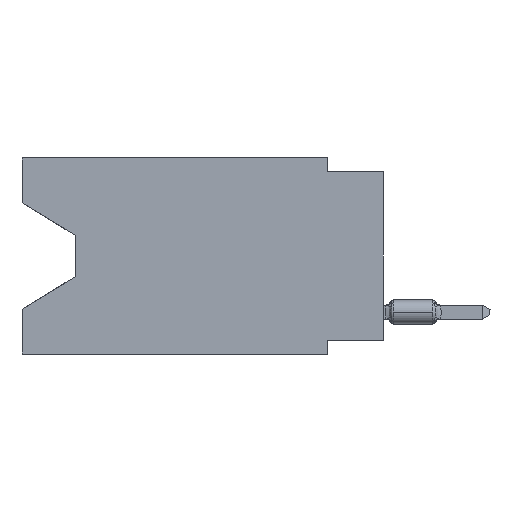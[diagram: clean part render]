
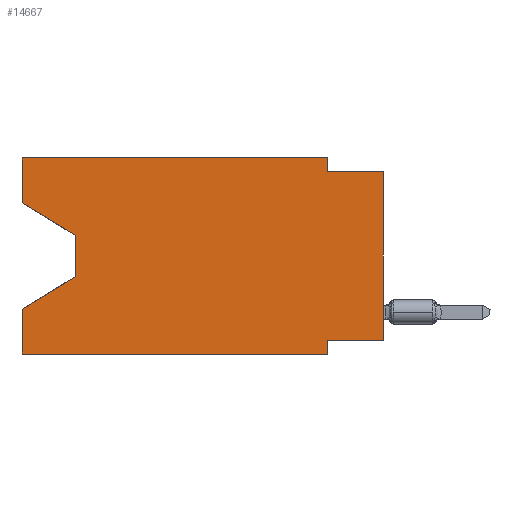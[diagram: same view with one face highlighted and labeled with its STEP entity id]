
A CAD part, left-side view. The second image highlights one B-rep face of the part: STEP entity #14667.
In plain terms, the highlighted planar face has unit normal (-1, 0, 0).
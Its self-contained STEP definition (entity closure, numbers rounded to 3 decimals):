
#1926 = EDGE_CURVE ( 'NONE', #49698, #31826, #39422, .T. ) ;
#3061 = EDGE_CURVE ( 'NONE', #45013, #55166, #20508, .T. ) ;
#3267 = VECTOR ( 'NONE', #7442, 1000. ) ;
#3288 = CARTESIAN_POINT ( 'NONE',  ( 0., 16.383, -2.038 ) ) ;
#3634 = ORIENTED_EDGE ( 'NONE', *, *, #1926, .T. ) ;
#4818 = LINE ( 'NONE', #38896, #38246 ) ;
#5095 = ORIENTED_EDGE ( 'NONE', *, *, #56931, .F. ) ;
#5235 = VECTOR ( 'NONE', #55082, 1000. ) ;
#5661 = DIRECTION ( 'NONE',  ( 0., 0., 1. ) ) ;
#6356 = LINE ( 'NONE', #35027, #21294 ) ;
#6646 = CARTESIAN_POINT ( 'NONE',  ( 0., 0., -0.635 ) ) ;
#7442 = DIRECTION ( 'NONE',  ( 0., -0.855, -0.519 ) ) ;
#9939 = ORIENTED_EDGE ( 'NONE', *, *, #15466, .F. ) ;
#11197 = CARTESIAN_POINT ( 'NONE',  ( 0., 16.383, -2.038 ) ) ;
#11342 = DIRECTION ( 'NONE',  ( 0., 0., -1. ) ) ;
#11903 = LINE ( 'NONE', #36718, #54903 ) ;
#12306 = DIRECTION ( 'NONE',  ( 0., 0., -1. ) ) ;
#12722 = VERTEX_POINT ( 'NONE', #15060 ) ;
#13015 = CARTESIAN_POINT ( 'NONE',  ( 0., 13.97, -3.505 ) ) ;
#13695 = VECTOR ( 'NONE', #55674, 1000. ) ;
#14220 = DIRECTION ( 'NONE',  ( 0., 0., -1. ) ) ;
#14667 = ADVANCED_FACE ( 'NONE', ( #22504 ), #56872, .F. ) ;
#14893 = CARTESIAN_POINT ( 'NONE',  ( 0., 13.97, -5.385 ) ) ;
#15060 = CARTESIAN_POINT ( 'NONE',  ( 0., 2.54, 0. ) ) ;
#15466 = EDGE_CURVE ( 'NONE', #27934, #31826, #26401, .T. ) ;
#16248 = LINE ( 'NONE', #59256, #5235 ) ;
#17161 = LINE ( 'NONE', #13015, #13695 ) ;
#17427 = VECTOR ( 'NONE', #5661, 1000. ) ;
#18581 = VECTOR ( 'NONE', #50697, 1000. ) ;
#19221 = EDGE_CURVE ( 'NONE', #59971, #35358, #51693, .T. ) ;
#19415 = ORIENTED_EDGE ( 'NONE', *, *, #21661, .T. ) ;
#19981 = ORIENTED_EDGE ( 'NONE', *, *, #3061, .T. ) ;
#20508 = LINE ( 'NONE', #31269, #18581 ) ;
#21294 = VECTOR ( 'NONE', #30865, 1000. ) ;
#21661 = EDGE_CURVE ( 'NONE', #35358, #45013, #17161, .T. ) ;
#22216 = LINE ( 'NONE', #41299, #54762 ) ;
#22504 = FACE_OUTER_BOUND ( 'NONE', #57175, .T. ) ;
#24315 = ORIENTED_EDGE ( 'NONE', *, *, #43636, .T. ) ;
#24591 = DIRECTION ( 'NONE',  ( 0., 0., 1. ) ) ;
#24799 = CARTESIAN_POINT ( 'NONE',  ( 0., 0., 0. ) ) ;
#24946 = VERTEX_POINT ( 'NONE', #50654 ) ;
#26094 = DIRECTION ( 'NONE',  ( 0., -1., 0. ) ) ;
#26401 = LINE ( 'NONE', #6646, #41769 ) ;
#27934 = VERTEX_POINT ( 'NONE', #52757 ) ;
#29991 = CARTESIAN_POINT ( 'NONE',  ( 0., 0., -8.255 ) ) ;
#30067 = CARTESIAN_POINT ( 'NONE',  ( 0., 2.54, -8.89 ) ) ;
#30627 = VECTOR ( 'NONE', #11342, 1000. ) ;
#30832 = VERTEX_POINT ( 'NONE', #30067 ) ;
#30865 = DIRECTION ( 'NONE',  ( 0., 0., 1. ) ) ;
#31107 = DIRECTION ( 'NONE',  ( 0., 1., 0. ) ) ;
#31269 = CARTESIAN_POINT ( 'NONE',  ( 0., 13.97, -5.385 ) ) ;
#31657 = CARTESIAN_POINT ( 'NONE',  ( 0., 13.97, -3.505 ) ) ;
#31826 = VERTEX_POINT ( 'NONE', #44076 ) ;
#31946 = DIRECTION ( 'NONE',  ( 0., -1., 0. ) ) ;
#32295 = CARTESIAN_POINT ( 'NONE',  ( 0., 16.383, -6.852 ) ) ;
#33554 = AXIS2_PLACEMENT_3D ( 'NONE', #51142, #56234, #12306 ) ;
#35027 = CARTESIAN_POINT ( 'NONE',  ( 0., 16.383, 0. ) ) ;
#35358 = VERTEX_POINT ( 'NONE', #31657 ) ;
#36171 = EDGE_CURVE ( 'NONE', #48090, #12722, #16248, .T. ) ;
#36718 = CARTESIAN_POINT ( 'NONE',  ( 0., 16.383, -8.89 ) ) ;
#37482 = LINE ( 'NONE', #43194, #45301 ) ;
#38246 = VECTOR ( 'NONE', #24591, 1000. ) ;
#38896 = CARTESIAN_POINT ( 'NONE',  ( 0., 16.383, 0. ) ) ;
#39422 = LINE ( 'NONE', #24799, #17427 ) ;
#41299 = CARTESIAN_POINT ( 'NONE',  ( 0., 0., -8.255 ) ) ;
#41602 = EDGE_CURVE ( 'NONE', #49698, #24946, #22216, .T. ) ;
#41769 = VECTOR ( 'NONE', #26094, 1000. ) ;
#42551 = ORIENTED_EDGE ( 'NONE', *, *, #45098, .F. ) ;
#43059 = EDGE_CURVE ( 'NONE', #59971, #48090, #6356, .T. ) ;
#43194 = CARTESIAN_POINT ( 'NONE',  ( 0., 2.54, 0. ) ) ;
#43636 = EDGE_CURVE ( 'NONE', #46102, #30832, #11903, .T. ) ;
#43863 = CARTESIAN_POINT ( 'NONE',  ( 0., 16.383, -8.89 ) ) ;
#44076 = CARTESIAN_POINT ( 'NONE',  ( 0., 0., -0.635 ) ) ;
#45013 = VERTEX_POINT ( 'NONE', #14893 ) ;
#45098 = EDGE_CURVE ( 'NONE', #24946, #30832, #59131, .T. ) ;
#45301 = VECTOR ( 'NONE', #14220, 1000. ) ;
#46102 = VERTEX_POINT ( 'NONE', #43863 ) ;
#48090 = VERTEX_POINT ( 'NONE', #49802 ) ;
#49698 = VERTEX_POINT ( 'NONE', #29991 ) ;
#49802 = CARTESIAN_POINT ( 'NONE',  ( 0., 16.383, 0. ) ) ;
#50654 = CARTESIAN_POINT ( 'NONE',  ( 0., 2.54, -8.255 ) ) ;
#50697 = DIRECTION ( 'NONE',  ( 0., 0.855, -0.519 ) ) ;
#51142 = CARTESIAN_POINT ( 'NONE',  ( 0., 16.383, 0. ) ) ;
#51693 = LINE ( 'NONE', #3288, #3267 ) ;
#52757 = CARTESIAN_POINT ( 'NONE',  ( 0., 2.54, -0.635 ) ) ;
#53708 = ORIENTED_EDGE ( 'NONE', *, *, #43059, .F. ) ;
#54339 = CARTESIAN_POINT ( 'NONE',  ( 0., 2.54, -8.89 ) ) ;
#54408 = ORIENTED_EDGE ( 'NONE', *, *, #36171, .F. ) ;
#54762 = VECTOR ( 'NONE', #31107, 1000. ) ;
#54903 = VECTOR ( 'NONE', #31946, 1000. ) ;
#55029 = ORIENTED_EDGE ( 'NONE', *, *, #56015, .F. ) ;
#55082 = DIRECTION ( 'NONE',  ( 0., -1., 0. ) ) ;
#55166 = VERTEX_POINT ( 'NONE', #32295 ) ;
#55674 = DIRECTION ( 'NONE',  ( 0., 0., -1. ) ) ;
#56015 = EDGE_CURVE ( 'NONE', #12722, #27934, #37482, .T. ) ;
#56234 = DIRECTION ( 'NONE',  ( 1., 0., 0. ) ) ;
#56872 = PLANE ( 'NONE',  #33554 ) ;
#56931 = EDGE_CURVE ( 'NONE', #46102, #55166, #4818, .T. ) ;
#57175 = EDGE_LOOP ( 'NONE', ( #59644, #19415, #19981, #5095, #24315, #42551, #58723, #3634, #9939, #55029, #54408, #53708 ) ) ;
#58723 = ORIENTED_EDGE ( 'NONE', *, *, #41602, .F. ) ;
#59131 = LINE ( 'NONE', #54339, #30627 ) ;
#59256 = CARTESIAN_POINT ( 'NONE',  ( 0., 16.383, 0. ) ) ;
#59644 = ORIENTED_EDGE ( 'NONE', *, *, #19221, .T. ) ;
#59971 = VERTEX_POINT ( 'NONE', #11197 ) ;
